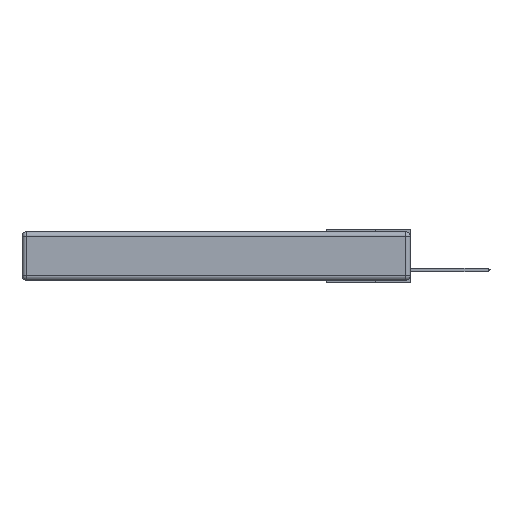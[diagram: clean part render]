
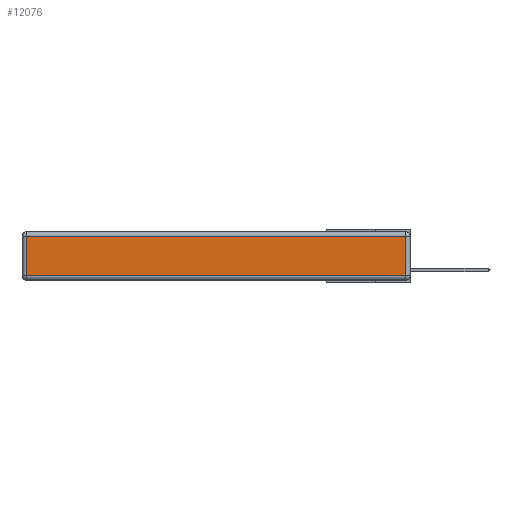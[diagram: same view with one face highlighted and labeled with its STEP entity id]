
A CAD part, left-side view. The second image highlights one B-rep face of the part: STEP entity #12076.
In plain terms, the highlighted planar face has unit normal (-1, 0, 0).
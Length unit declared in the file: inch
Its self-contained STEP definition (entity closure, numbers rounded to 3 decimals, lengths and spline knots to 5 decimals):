
#220 = LINE ( 'NONE', #5265, #15283 ) ;
#331 = DIRECTION ( 'NONE',  ( 0., 1., 0. ) ) ;
#476 = LINE ( 'NONE', #15436, #8439 ) ;
#1049 = CARTESIAN_POINT ( 'NONE',  ( 0., 2.72, -0.03 ) ) ;
#1790 = CARTESIAN_POINT ( 'NONE',  ( 0., 0.03, -0.313 ) ) ;
#1938 = LINE ( 'NONE', #11990, #12488 ) ;
#2383 = ORIENTED_EDGE ( 'NONE', *, *, #12964, .T. ) ;
#2552 = CARTESIAN_POINT ( 'NONE',  ( 0., 2.72, -0.313 ) ) ;
#2597 = EDGE_CURVE ( 'NONE', #4817, #6068, #1938, .T. ) ;
#3097 = VERTEX_POINT ( 'NONE', #3667 ) ;
#3179 = DIRECTION ( 'NONE',  ( -1., 0., 0. ) ) ;
#3667 = CARTESIAN_POINT ( 'NONE',  ( 0., 0.03, -0.03 ) ) ;
#3953 = DIRECTION ( 'NONE',  ( 0., 0., -1. ) ) ;
#4416 = ORIENTED_EDGE ( 'NONE', *, *, #6686, .T. ) ;
#4500 = DIRECTION ( 'NONE',  ( 0., -1., 0. ) ) ;
#4817 = VERTEX_POINT ( 'NONE', #2552 ) ;
#5265 = CARTESIAN_POINT ( 'NONE',  ( 0., 0.03, -0.343 ) ) ;
#5378 = DIRECTION ( 'NONE',  ( 0., 0., 1. ) ) ;
#5811 = VECTOR ( 'NONE', #3953, 39.37008 ) ;
#5833 = ORIENTED_EDGE ( 'NONE', *, *, #6775, .T. ) ;
#6068 = VERTEX_POINT ( 'NONE', #1790 ) ;
#6383 = CARTESIAN_POINT ( 'NONE',  ( 0., 2.72, -0.343 ) ) ;
#6686 = EDGE_CURVE ( 'NONE', #13522, #4817, #12111, .T. ) ;
#6692 = EDGE_LOOP ( 'NONE', ( #11003, #5833, #2383, #4416 ) ) ;
#6775 = EDGE_CURVE ( 'NONE', #6068, #3097, #220, .T. ) ;
#6878 = AXIS2_PLACEMENT_3D ( 'NONE', #9426, #3179, #11909 ) ;
#8439 = VECTOR ( 'NONE', #331, 39.37008 ) ;
#9426 = CARTESIAN_POINT ( 'NONE',  ( 0., 0., -0.343 ) ) ;
#9607 = FACE_OUTER_BOUND ( 'NONE', #6692, .T. ) ;
#11003 = ORIENTED_EDGE ( 'NONE', *, *, #2597, .T. ) ;
#11909 = DIRECTION ( 'NONE',  ( 0., 0., 1. ) ) ;
#11990 = CARTESIAN_POINT ( 'NONE',  ( 0., 0., -0.313 ) ) ;
#12076 = ADVANCED_FACE ( 'NONE', ( #9607 ), #14478, .T. ) ;
#12111 = LINE ( 'NONE', #6383, #5811 ) ;
#12488 = VECTOR ( 'NONE', #4500, 39.37008 ) ;
#12964 = EDGE_CURVE ( 'NONE', #3097, #13522, #476, .T. ) ;
#13522 = VERTEX_POINT ( 'NONE', #1049 ) ;
#14478 = PLANE ( 'NONE',  #6878 ) ;
#15283 = VECTOR ( 'NONE', #5378, 39.37008 ) ;
#15436 = CARTESIAN_POINT ( 'NONE',  ( 0., 2.75, -0.03 ) ) ;
